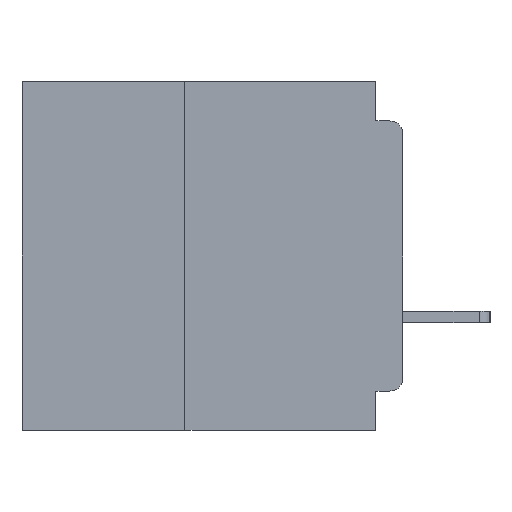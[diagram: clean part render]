
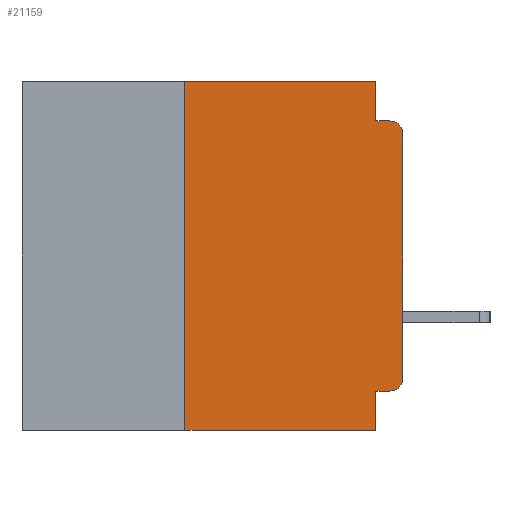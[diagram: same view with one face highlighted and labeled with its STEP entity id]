
A CAD part, left-side view. The second image highlights one B-rep face of the part: STEP entity #21159.
In plain terms, the highlighted planar face has unit normal (-1, 0, 0).
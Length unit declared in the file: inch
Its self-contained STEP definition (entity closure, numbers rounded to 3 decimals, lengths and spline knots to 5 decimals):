
#425 = ORIENTED_EDGE ( 'NONE', *, *, #11138, .T. ) ;
#733 = LINE ( 'NONE', #36485, #36985 ) ;
#1147 = DIRECTION ( 'NONE',  ( -1., 0., 0. ) ) ;
#1897 = DIRECTION ( 'NONE',  ( 0., 0., -1. ) ) ;
#2030 = ORIENTED_EDGE ( 'NONE', *, *, #38969, .F. ) ;
#2555 = EDGE_CURVE ( 'NONE', #34150, #44550, #45351, .T. ) ;
#3369 = ORIENTED_EDGE ( 'NONE', *, *, #13194, .T. ) ;
#5137 = VERTEX_POINT ( 'NONE', #35019 ) ;
#5741 = VECTOR ( 'NONE', #31727, 39.37008 ) ;
#6876 = EDGE_CURVE ( 'NONE', #8120, #27716, #43059, .T. ) ;
#7071 = ORIENTED_EDGE ( 'NONE', *, *, #43934, .F. ) ;
#7369 = LINE ( 'NONE', #32604, #15582 ) ;
#7531 = EDGE_CURVE ( 'NONE', #42583, #34280, #7369, .T. ) ;
#8068 = AXIS2_PLACEMENT_3D ( 'NONE', #22197, #1147, #25713 ) ;
#8120 = VERTEX_POINT ( 'NONE', #9735 ) ;
#8266 = PLANE ( 'NONE',  #25934 ) ;
#9735 = CARTESIAN_POINT ( 'NONE',  ( 0., 0.25, 0. ) ) ;
#11138 = EDGE_CURVE ( 'NONE', #27720, #25206, #29092, .T. ) ;
#12181 = VECTOR ( 'NONE', #30259, 39.37008 ) ;
#12376 = VECTOR ( 'NONE', #30492, 39.37008 ) ;
#12414 = CARTESIAN_POINT ( 'NONE',  ( 0., 0.25, -0.4 ) ) ;
#12822 = CARTESIAN_POINT ( 'NONE',  ( 0., 0., 0. ) ) ;
#13194 = EDGE_CURVE ( 'NONE', #44550, #27720, #32177, .T. ) ;
#13265 = LINE ( 'NONE', #26698, #12181 ) ;
#13333 = CARTESIAN_POINT ( 'NONE',  ( 0., 0.015, -0.045 ) ) ;
#13750 = CARTESIAN_POINT ( 'NONE',  ( 0., 0., -0.06 ) ) ;
#13756 = ORIENTED_EDGE ( 'NONE', *, *, #6876, .F. ) ;
#14014 = ORIENTED_EDGE ( 'NONE', *, *, #14072, .F. ) ;
#14072 = EDGE_CURVE ( 'NONE', #19786, #25206, #733, .T. ) ;
#15307 = DIRECTION ( 'NONE',  ( 0., 0., -1. ) ) ;
#15582 = VECTOR ( 'NONE', #21985, 39.37008 ) ;
#17092 = VECTOR ( 'NONE', #34067, 39.37008 ) ;
#17557 = CARTESIAN_POINT ( 'NONE',  ( 0., 0.437, 0. ) ) ;
#19459 = DIRECTION ( 'NONE',  ( 0., 0., 1. ) ) ;
#19786 = VERTEX_POINT ( 'NONE', #39181 ) ;
#21159 = ADVANCED_FACE ( 'NONE', ( #44968 ), #8266, .F. ) ;
#21985 = DIRECTION ( 'NONE',  ( 0., -1., 0. ) ) ;
#22197 = CARTESIAN_POINT ( 'NONE',  ( 0., 0.015, -0.06 ) ) ;
#22957 = DIRECTION ( 'NONE',  ( -1., 0., 0. ) ) ;
#23303 = LINE ( 'NONE', #27710, #31563 ) ;
#23623 = CARTESIAN_POINT ( 'NONE',  ( 0., 0., -0.355 ) ) ;
#24027 = EDGE_CURVE ( 'NONE', #42583, #8120, #40397, .T. ) ;
#25139 = AXIS2_PLACEMENT_3D ( 'NONE', #43875, #22957, #1897 ) ;
#25206 = VERTEX_POINT ( 'NONE', #13333 ) ;
#25713 = DIRECTION ( 'NONE',  ( 0., 0., -1. ) ) ;
#25934 = AXIS2_PLACEMENT_3D ( 'NONE', #32850, #36352, #15307 ) ;
#26698 = CARTESIAN_POINT ( 'NONE',  ( 0., 0.031, -0.4 ) ) ;
#26791 = ORIENTED_EDGE ( 'NONE', *, *, #24027, .F. ) ;
#27682 = EDGE_LOOP ( 'NONE', ( #3369, #425, #14014, #37406, #13756, #26791, #30912, #2030, #7071, #43279 ) ) ;
#27710 = CARTESIAN_POINT ( 'NONE',  ( 0., 0.031, 0. ) ) ;
#27716 = VERTEX_POINT ( 'NONE', #34792 ) ;
#27720 = VERTEX_POINT ( 'NONE', #13750 ) ;
#29092 = CIRCLE ( 'NONE', #8068, 0.015 ) ;
#30259 = DIRECTION ( 'NONE',  ( 0., 0., -1. ) ) ;
#30492 = DIRECTION ( 'NONE',  ( 0., 0., 1. ) ) ;
#30912 = ORIENTED_EDGE ( 'NONE', *, *, #7531, .T. ) ;
#31145 = VECTOR ( 'NONE', #19459, 39.37008 ) ;
#31255 = DIRECTION ( 'NONE',  ( 0., 0., -1. ) ) ;
#31563 = VECTOR ( 'NONE', #31255, 39.37008 ) ;
#31727 = DIRECTION ( 'NONE',  ( 0., -1., 0. ) ) ;
#32177 = LINE ( 'NONE', #12822, #12376 ) ;
#32604 = CARTESIAN_POINT ( 'NONE',  ( 0., 0.437, -0.4 ) ) ;
#32850 = CARTESIAN_POINT ( 'NONE',  ( 0., 0.437, 0. ) ) ;
#33566 = CARTESIAN_POINT ( 'NONE',  ( 0., 0.25, -0.4 ) ) ;
#34067 = DIRECTION ( 'NONE',  ( 0., 1., 0. ) ) ;
#34150 = VERTEX_POINT ( 'NONE', #39931 ) ;
#34280 = VERTEX_POINT ( 'NONE', #37043 ) ;
#34477 = CARTESIAN_POINT ( 'NONE',  ( 0., 0., -0.34 ) ) ;
#34792 = CARTESIAN_POINT ( 'NONE',  ( 0., 0.031, 0. ) ) ;
#35019 = CARTESIAN_POINT ( 'NONE',  ( 0., 0.031, -0.355 ) ) ;
#35821 = LINE ( 'NONE', #23623, #17092 ) ;
#36352 = DIRECTION ( 'NONE',  ( 1., 0., 0. ) ) ;
#36485 = CARTESIAN_POINT ( 'NONE',  ( 0., 0., -0.045 ) ) ;
#36985 = VECTOR ( 'NONE', #39969, 39.37008 ) ;
#37043 = CARTESIAN_POINT ( 'NONE',  ( 0., 0.031, -0.4 ) ) ;
#37406 = ORIENTED_EDGE ( 'NONE', *, *, #42772, .F. ) ;
#38969 = EDGE_CURVE ( 'NONE', #5137, #34280, #13265, .T. ) ;
#39181 = CARTESIAN_POINT ( 'NONE',  ( 0., 0.031, -0.045 ) ) ;
#39931 = CARTESIAN_POINT ( 'NONE',  ( 0., 0.015, -0.355 ) ) ;
#39969 = DIRECTION ( 'NONE',  ( 0., -1., 0. ) ) ;
#40397 = LINE ( 'NONE', #12414, #31145 ) ;
#42583 = VERTEX_POINT ( 'NONE', #33566 ) ;
#42772 = EDGE_CURVE ( 'NONE', #27716, #19786, #23303, .T. ) ;
#43059 = LINE ( 'NONE', #17557, #5741 ) ;
#43279 = ORIENTED_EDGE ( 'NONE', *, *, #2555, .T. ) ;
#43875 = CARTESIAN_POINT ( 'NONE',  ( 0., 0.015, -0.34 ) ) ;
#43934 = EDGE_CURVE ( 'NONE', #34150, #5137, #35821, .T. ) ;
#44550 = VERTEX_POINT ( 'NONE', #34477 ) ;
#44968 = FACE_OUTER_BOUND ( 'NONE', #27682, .T. ) ;
#45351 = CIRCLE ( 'NONE', #25139, 0.015 ) ;
